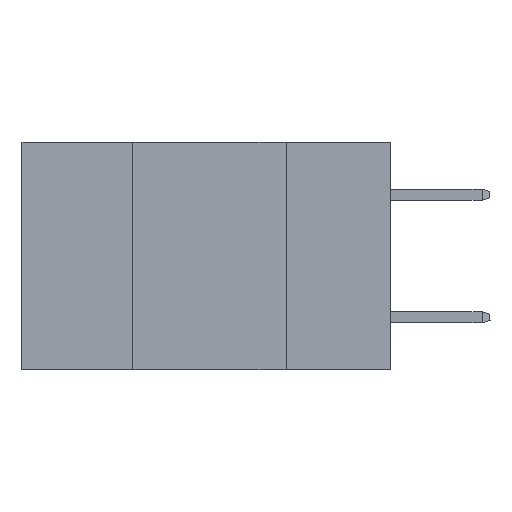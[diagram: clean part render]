
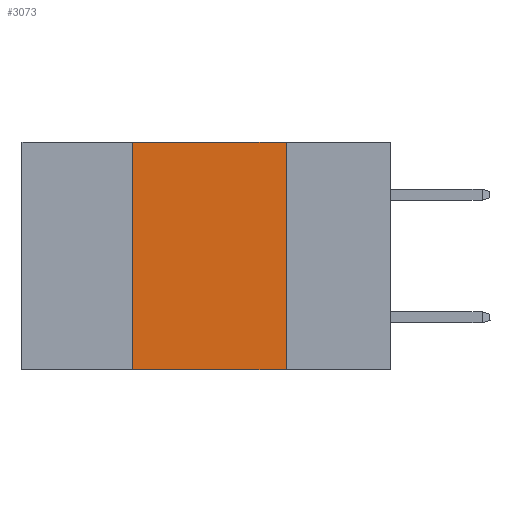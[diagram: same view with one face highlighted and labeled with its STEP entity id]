
A CAD part, left-side view. The second image highlights one B-rep face of the part: STEP entity #3073.
In plain terms, the highlighted planar face has unit normal (-1, 0, 0).
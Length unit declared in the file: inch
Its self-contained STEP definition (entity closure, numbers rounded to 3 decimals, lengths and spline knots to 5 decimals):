
#323 = FACE_OUTER_BOUND ( 'NONE', #18565, .T. ) ;
#399 = CARTESIAN_POINT ( 'NONE',  ( 0., 0.17, 0. ) ) ;
#1219 = VECTOR ( 'NONE', #11458, 39.37008 ) ;
#3073 = ADVANCED_FACE ( 'NONE', ( #323 ), #8924, .F. ) ;
#4827 = EDGE_CURVE ( 'NONE', #21092, #7517, #6558, .T. ) ;
#5776 = CARTESIAN_POINT ( 'NONE',  ( 0., 0.6, -0.37 ) ) ;
#5999 = EDGE_CURVE ( 'NONE', #8613, #7517, #6808, .T. ) ;
#6558 = LINE ( 'NONE', #19188, #11680 ) ;
#6808 = LINE ( 'NONE', #5776, #25552 ) ;
#7356 = CARTESIAN_POINT ( 'NONE',  ( 0., 0.42, -0.37 ) ) ;
#7517 = VERTEX_POINT ( 'NONE', #12710 ) ;
#7982 = VECTOR ( 'NONE', #21868, 39.37008 ) ;
#8613 = VERTEX_POINT ( 'NONE', #7356 ) ;
#8924 = PLANE ( 'NONE',  #17167 ) ;
#9186 = DIRECTION ( 'NONE',  ( 0., 0., -1. ) ) ;
#9191 = ORIENTED_EDGE ( 'NONE', *, *, #5999, .T. ) ;
#10826 = LINE ( 'NONE', #11543, #1219 ) ;
#11458 = DIRECTION ( 'NONE',  ( 0., 0., 1. ) ) ;
#11501 = LINE ( 'NONE', #21607, #7982 ) ;
#11543 = CARTESIAN_POINT ( 'NONE',  ( 0., 0.42, 0. ) ) ;
#11680 = VECTOR ( 'NONE', #23644, 39.37008 ) ;
#12018 = DIRECTION ( 'NONE',  ( 0., -1., 0. ) ) ;
#12710 = CARTESIAN_POINT ( 'NONE',  ( 0., 0.17, -0.37 ) ) ;
#17167 = AXIS2_PLACEMENT_3D ( 'NONE', #23343, #25715, #9186 ) ;
#18533 = ORIENTED_EDGE ( 'NONE', *, *, #4827, .F. ) ;
#18565 = EDGE_LOOP ( 'NONE', ( #18533, #22052, #24383, #9191 ) ) ;
#19188 = CARTESIAN_POINT ( 'NONE',  ( 0., 0.17, 0. ) ) ;
#19479 = CARTESIAN_POINT ( 'NONE',  ( 0., 0.42, 0. ) ) ;
#21092 = VERTEX_POINT ( 'NONE', #399 ) ;
#21607 = CARTESIAN_POINT ( 'NONE',  ( 0., 0.6, 0. ) ) ;
#21868 = DIRECTION ( 'NONE',  ( 0., -1., 0. ) ) ;
#22052 = ORIENTED_EDGE ( 'NONE', *, *, #25072, .F. ) ;
#23343 = CARTESIAN_POINT ( 'NONE',  ( 0., 0.6, 0. ) ) ;
#23417 = VERTEX_POINT ( 'NONE', #19479 ) ;
#23644 = DIRECTION ( 'NONE',  ( 0., 0., -1. ) ) ;
#24383 = ORIENTED_EDGE ( 'NONE', *, *, #25616, .F. ) ;
#25072 = EDGE_CURVE ( 'NONE', #23417, #21092, #11501, .T. ) ;
#25552 = VECTOR ( 'NONE', #12018, 39.37008 ) ;
#25616 = EDGE_CURVE ( 'NONE', #8613, #23417, #10826, .T. ) ;
#25715 = DIRECTION ( 'NONE',  ( 1., 0., 0. ) ) ;
